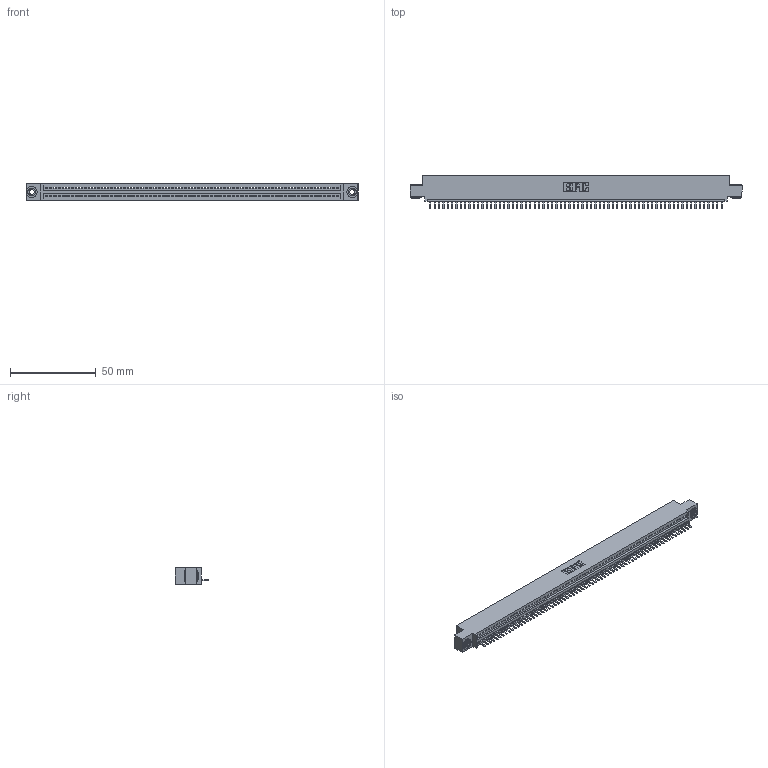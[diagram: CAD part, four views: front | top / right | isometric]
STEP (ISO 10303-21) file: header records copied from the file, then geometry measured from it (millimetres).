
FILE_DESCRIPTION (( 'STEP AP203' ), '1' );
FILE_NAME ('395-068-520-403.STEP', '2019-10-25T14:42:22', ( '' ), ( '' ), 'SwSTEP 2.0', 'SolidWorks 2016', '' );
FILE_SCHEMA (( 'CONFIG_CONTROL_DESIGN' ));
Length unit declared in the file: inch
Products named in the file (4): 395-068-520-403; 345 Part_0.110 Offset - 0.156 Dia-TH; 345-292-001_345-293-120; 345-250-002_345-250-002-102
Assembly tree (71 placements, depth 2):
  395-068-520-403
    345 Part_0.110 Offset - 0.156 Dia-TH
    345-292-001_345-293-120  x68
    345-250-002_345-250-002-102  x2
Bounding box: 193.93 x 19.68 x 9.4 mm (x, y, z)
Volume: 18383 mm3; surface area: 24439.1 mm2
Topology: 71 solids, 71 shells, 4384 faces, 12941 edges, 8442 vertices
Faces by surface type: plane 2950, cylinder 1426, cone 8
Entity records: 48574 total; most frequent: CARTESIAN_POINT 8403, ORIENTED_EDGE 8386, DIRECTION 7319, EDGE_CURVE 4193, VECTOR 3761, LINE 3761, VERTEX_POINT 2790, AXIS2_PLACEMENT_3D 1779
